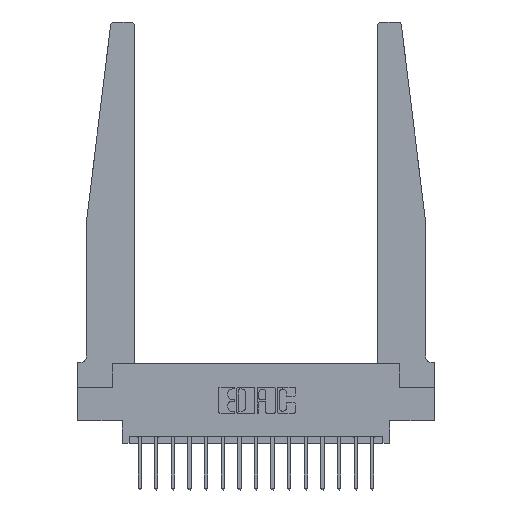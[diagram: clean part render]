
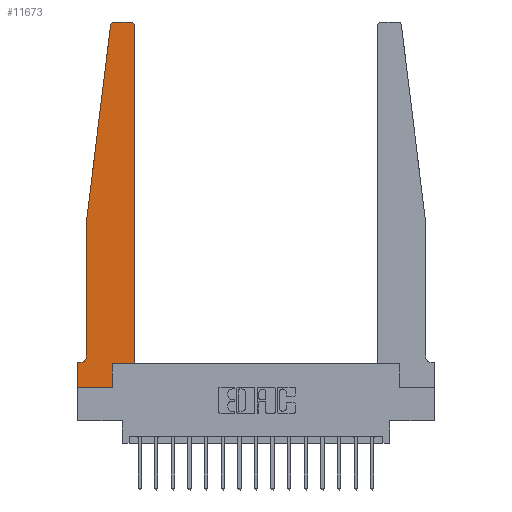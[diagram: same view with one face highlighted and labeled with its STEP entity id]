
A CAD part, top view. The second image highlights one B-rep face of the part: STEP entity #11673.
In plain terms, the highlighted planar face has unit normal (0, 0, 1).
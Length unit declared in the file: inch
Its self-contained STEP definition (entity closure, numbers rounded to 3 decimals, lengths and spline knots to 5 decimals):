
#70 = VECTOR ( 'NONE', #5077, 39.37008 ) ;
#542 = LINE ( 'NONE', #11011, #5920 ) ;
#568 = CARTESIAN_POINT ( 'NONE',  ( 0.27653, 2.72, 0.37 ) ) ;
#790 = EDGE_CURVE ( 'NONE', #17378, #5239, #17578, .T. ) ;
#808 = DIRECTION ( 'NONE',  ( -1., 0., 0. ) ) ;
#1430 = VECTOR ( 'NONE', #10297, 39.37008 ) ;
#1527 = CARTESIAN_POINT ( 'NONE',  ( 0., 0., 0.37 ) ) ;
#1542 = DIRECTION ( 'NONE',  ( 1., 0., 0. ) ) ;
#1937 = VERTEX_POINT ( 'NONE', #2377 ) ;
#2232 = DIRECTION ( 'NONE',  ( 0., 0., -1. ) ) ;
#2250 = VECTOR ( 'NONE', #1542, 39.37008 ) ;
#2377 = CARTESIAN_POINT ( 'NONE',  ( 0.425, 2.72, 0.37 ) ) ;
#2441 = CARTESIAN_POINT ( 'NONE',  ( 0.24675, 2.72367, 0.37 ) ) ;
#2664 = ORIENTED_EDGE ( 'NONE', *, *, #6930, .T. ) ;
#2699 = LINE ( 'NONE', #18546, #2250 ) ;
#2839 = ORIENTED_EDGE ( 'NONE', *, *, #9597, .T. ) ;
#2846 = EDGE_CURVE ( 'NONE', #8576, #11151, #10949, .T. ) ;
#3562 = AXIS2_PLACEMENT_3D ( 'NONE', #4923, #9746, #17066 ) ;
#3611 = FACE_OUTER_BOUND ( 'NONE', #18030, .T. ) ;
#3809 = EDGE_CURVE ( 'NONE', #13438, #1937, #4801, .T. ) ;
#4037 = DIRECTION ( 'NONE',  ( -0.122, -0.992, 0. ) ) ;
#4054 = VECTOR ( 'NONE', #5888, 39.37008 ) ;
#4156 = CARTESIAN_POINT ( 'NONE',  ( 0., 0.1875, 0.37 ) ) ;
#4276 = DIRECTION ( 'NONE',  ( 1., 0., 0. ) ) ;
#4416 = VERTEX_POINT ( 'NONE', #15372 ) ;
#4443 = EDGE_CURVE ( 'NONE', #7857, #4416, #10905, .T. ) ;
#4708 = CIRCLE ( 'NONE', #7726, 0.03 ) ;
#4801 = LINE ( 'NONE', #10570, #70 ) ;
#4902 = ORIENTED_EDGE ( 'NONE', *, *, #2846, .T. ) ;
#4923 = CARTESIAN_POINT ( 'NONE',  ( 0., 0.1875, 0.37 ) ) ;
#5077 = DIRECTION ( 'NONE',  ( 0., 1., 0. ) ) ;
#5086 = CARTESIAN_POINT ( 'NONE',  ( 0.395, 2.72, 0.37 ) ) ;
#5189 = DIRECTION ( 'NONE',  ( 1., 0., 0. ) ) ;
#5239 = VERTEX_POINT ( 'NONE', #10569 ) ;
#5460 = ORIENTED_EDGE ( 'NONE', *, *, #8031, .T. ) ;
#5705 = LINE ( 'NONE', #1527, #12052 ) ;
#5736 = VECTOR ( 'NONE', #4037, 39.37008 ) ;
#5819 = ORIENTED_EDGE ( 'NONE', *, *, #13769, .T. ) ;
#5876 = CARTESIAN_POINT ( 'NONE',  ( 0.065, 0.1875, 0.37 ) ) ;
#5882 = ORIENTED_EDGE ( 'NONE', *, *, #790, .T. ) ;
#5888 = DIRECTION ( 'NONE',  ( -1., 0., 0. ) ) ;
#5920 = VECTOR ( 'NONE', #6593, 39.37008 ) ;
#5976 = ORIENTED_EDGE ( 'NONE', *, *, #4443, .T. ) ;
#6022 = CARTESIAN_POINT ( 'NONE',  ( 0.015, 0.1875, 0.37 ) ) ;
#6593 = DIRECTION ( 'NONE',  ( 0., -1., 0. ) ) ;
#6930 = EDGE_CURVE ( 'NONE', #15493, #13438, #2699, .T. ) ;
#7105 = CARTESIAN_POINT ( 'NONE',  ( 0.25, 2.75, 0.37 ) ) ;
#7451 = CARTESIAN_POINT ( 'NONE',  ( 0.395, 2.75, 0.37 ) ) ;
#7567 = EDGE_CURVE ( 'NONE', #11151, #7857, #10409, .T. ) ;
#7628 = EDGE_CURVE ( 'NONE', #5239, #13865, #4708, .T. ) ;
#7661 = CARTESIAN_POINT ( 'NONE',  ( 0.2605, 0.18, 0.37 ) ) ;
#7726 = AXIS2_PLACEMENT_3D ( 'NONE', #568, #16773, #5189 ) ;
#7857 = VERTEX_POINT ( 'NONE', #4156 ) ;
#8004 = CARTESIAN_POINT ( 'NONE',  ( 0.015, 0.2375, 0.37 ) ) ;
#8031 = EDGE_CURVE ( 'NONE', #16864, #8576, #542, .T. ) ;
#8042 = PLANE ( 'NONE',  #3562 ) ;
#8104 = CIRCLE ( 'NONE', #17818, 0.03 ) ;
#8576 = VERTEX_POINT ( 'NONE', #9107 ) ;
#8887 = CARTESIAN_POINT ( 'NONE',  ( 0.2605, 0.18, 0.37 ) ) ;
#8941 = CARTESIAN_POINT ( 'NONE',  ( 0.2605, 0., 0.37 ) ) ;
#9107 = CARTESIAN_POINT ( 'NONE',  ( 0.065, 0.2375, 0.37 ) ) ;
#9180 = VECTOR ( 'NONE', #18261, 39.37008 ) ;
#9424 = ORIENTED_EDGE ( 'NONE', *, *, #7628, .T. ) ;
#9597 = EDGE_CURVE ( 'NONE', #9728, #15493, #14742, .T. ) ;
#9728 = VERTEX_POINT ( 'NONE', #8941 ) ;
#9746 = DIRECTION ( 'NONE',  ( 0., 0., 1. ) ) ;
#10297 = DIRECTION ( 'NONE',  ( 0., 1., 0. ) ) ;
#10409 = LINE ( 'NONE', #5876, #18354 ) ;
#10569 = CARTESIAN_POINT ( 'NONE',  ( 0.27653, 2.75, 0.37 ) ) ;
#10570 = CARTESIAN_POINT ( 'NONE',  ( 0.425, 0.18, 0.37 ) ) ;
#10905 = LINE ( 'NONE', #15271, #9180 ) ;
#10949 = CIRCLE ( 'NONE', #14564, 0.05 ) ;
#11011 = CARTESIAN_POINT ( 'NONE',  ( 0.065, 1.25, 0.37 ) ) ;
#11151 = VERTEX_POINT ( 'NONE', #6022 ) ;
#11665 = CARTESIAN_POINT ( 'NONE',  ( 0.065, 1.25, 0.37 ) ) ;
#11673 = ADVANCED_FACE ( 'NONE', ( #3611 ), #8042, .T. ) ;
#12052 = VECTOR ( 'NONE', #4276, 39.37008 ) ;
#12083 = EDGE_CURVE ( 'NONE', #1937, #17378, #8104, .T. ) ;
#12536 = ORIENTED_EDGE ( 'NONE', *, *, #3809, .T. ) ;
#12802 = ORIENTED_EDGE ( 'NONE', *, *, #12083, .T. ) ;
#13438 = VERTEX_POINT ( 'NONE', #15772 ) ;
#13474 = ORIENTED_EDGE ( 'NONE', *, *, #13884, .T. ) ;
#13769 = EDGE_CURVE ( 'NONE', #4416, #9728, #5705, .T. ) ;
#13865 = VERTEX_POINT ( 'NONE', #2441 ) ;
#13884 = EDGE_CURVE ( 'NONE', #13865, #16864, #16673, .T. ) ;
#14564 = AXIS2_PLACEMENT_3D ( 'NONE', #8004, #2232, #808 ) ;
#14742 = LINE ( 'NONE', #8887, #1430 ) ;
#14749 = DIRECTION ( 'NONE',  ( 1., 0., 0. ) ) ;
#15271 = CARTESIAN_POINT ( 'NONE',  ( 0., 0., 0.37 ) ) ;
#15372 = CARTESIAN_POINT ( 'NONE',  ( 0., 0., 0.37 ) ) ;
#15493 = VERTEX_POINT ( 'NONE', #7661 ) ;
#15772 = CARTESIAN_POINT ( 'NONE',  ( 0.425, 0.18, 0.37 ) ) ;
#16213 = DIRECTION ( 'NONE',  ( -1., 0., 0. ) ) ;
#16673 = LINE ( 'NONE', #17337, #5736 ) ;
#16773 = DIRECTION ( 'NONE',  ( 0., 0., 1. ) ) ;
#16864 = VERTEX_POINT ( 'NONE', #11665 ) ;
#17066 = DIRECTION ( 'NONE',  ( 1., 0., 0. ) ) ;
#17337 = CARTESIAN_POINT ( 'NONE',  ( 0.065, 1.25, 0.37 ) ) ;
#17378 = VERTEX_POINT ( 'NONE', #7451 ) ;
#17578 = LINE ( 'NONE', #7105, #4054 ) ;
#17818 = AXIS2_PLACEMENT_3D ( 'NONE', #5086, #17920, #14749 ) ;
#17920 = DIRECTION ( 'NONE',  ( 0., 0., 1. ) ) ;
#18030 = EDGE_LOOP ( 'NONE', ( #5882, #9424, #13474, #5460, #4902, #18437, #5976, #5819, #2839, #2664, #12536, #12802 ) ) ;
#18261 = DIRECTION ( 'NONE',  ( 0., -1., 0. ) ) ;
#18354 = VECTOR ( 'NONE', #16213, 39.37008 ) ;
#18437 = ORIENTED_EDGE ( 'NONE', *, *, #7567, .T. ) ;
#18546 = CARTESIAN_POINT ( 'NONE',  ( 0.425, 0.18, 0.37 ) ) ;
